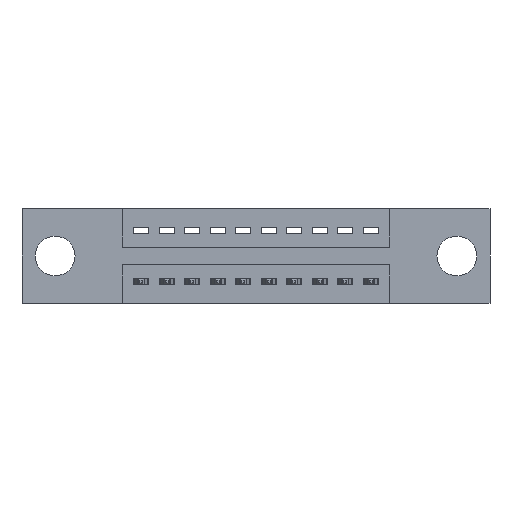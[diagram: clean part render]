
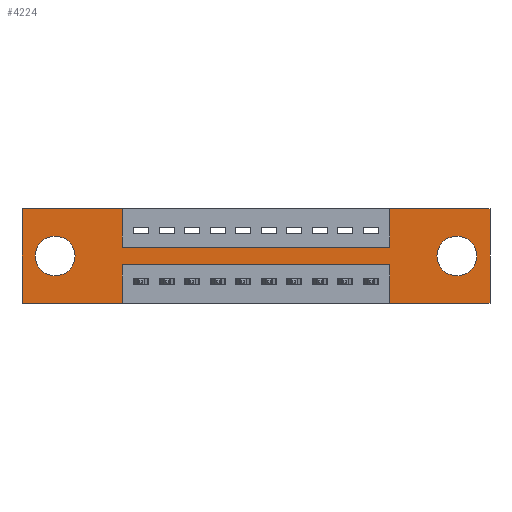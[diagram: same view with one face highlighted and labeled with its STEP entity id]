
A CAD part, front view. The second image highlights one B-rep face of the part: STEP entity #4224.
In plain terms, the highlighted planar face has unit normal (0, -1, 0).
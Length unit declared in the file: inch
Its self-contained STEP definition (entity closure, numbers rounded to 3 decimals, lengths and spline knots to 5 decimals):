
#251 = ORIENTED_EDGE ( 'NONE', *, *, #331, .F. ) ;
#302 = EDGE_CURVE ( 'NONE', #4691, #10908, #1327, .T. ) ;
#331 = EDGE_CURVE ( 'NONE', #7108, #2390, #3568, .T. ) ;
#503 = VECTOR ( 'NONE', #3563, 39.37008 ) ;
#579 = CARTESIAN_POINT ( 'NONE',  ( 0.3925, 0., -0.22 ) ) ;
#638 = CIRCLE ( 'NONE', #8570, 0.078 ) ;
#676 = EDGE_CURVE ( 'NONE', #3560, #1335, #5312, .T. ) ;
#864 = LINE ( 'NONE', #6454, #5596 ) ;
#876 = ORIENTED_EDGE ( 'NONE', *, *, #302, .T. ) ;
#935 = CARTESIAN_POINT ( 'NONE',  ( 0.13, 0., -0.185 ) ) ;
#1036 = VECTOR ( 'NONE', #4427, 39.37008 ) ;
#1044 = EDGE_CURVE ( 'NONE', #5193, #8139, #10566, .T. ) ;
#1082 = VECTOR ( 'NONE', #11482, 39.37008 ) ;
#1116 = EDGE_CURVE ( 'NONE', #2390, #2133, #864, .T. ) ;
#1207 = CIRCLE ( 'NONE', #10180, 0.078 ) ;
#1274 = FACE_BOUND ( 'NONE', #7116, .T. ) ;
#1327 = CIRCLE ( 'NONE', #3244, 0.078 ) ;
#1335 = VERTEX_POINT ( 'NONE', #3687 ) ;
#1365 = VECTOR ( 'NONE', #3258, 39.37008 ) ;
#1405 = DIRECTION ( 'NONE',  ( 0., 1., 0. ) ) ;
#1567 = FACE_BOUND ( 'NONE', #4058, .T. ) ;
#1664 = CARTESIAN_POINT ( 'NONE',  ( 1.835, 0., 0. ) ) ;
#1784 = CARTESIAN_POINT ( 'NONE',  ( 0.3925, 0., -0.15 ) ) ;
#1871 = DIRECTION ( 'NONE',  ( 0., 0., 1. ) ) ;
#2133 = VERTEX_POINT ( 'NONE', #1784 ) ;
#2157 = CARTESIAN_POINT ( 'NONE',  ( 0., 0., 0. ) ) ;
#2176 = CARTESIAN_POINT ( 'NONE',  ( 0., 0., 0. ) ) ;
#2212 = CARTESIAN_POINT ( 'NONE',  ( 0.3925, 0., -0.37 ) ) ;
#2390 = VERTEX_POINT ( 'NONE', #10811 ) ;
#2412 = EDGE_CURVE ( 'NONE', #10908, #4691, #8534, .T. ) ;
#2504 = ORIENTED_EDGE ( 'NONE', *, *, #10839, .F. ) ;
#2682 = VECTOR ( 'NONE', #3116, 39.37008 ) ;
#2815 = VECTOR ( 'NONE', #5090, 39.37008 ) ;
#2950 = ORIENTED_EDGE ( 'NONE', *, *, #1116, .F. ) ;
#2960 = VERTEX_POINT ( 'NONE', #6413 ) ;
#3116 = DIRECTION ( 'NONE',  ( 1., 0., 0. ) ) ;
#3244 = AXIS2_PLACEMENT_3D ( 'NONE', #4692, #5480, #7324 ) ;
#3258 = DIRECTION ( 'NONE',  ( 0., 0., 1. ) ) ;
#3499 = VERTEX_POINT ( 'NONE', #2212 ) ;
#3560 = VERTEX_POINT ( 'NONE', #1664 ) ;
#3563 = DIRECTION ( 'NONE',  ( 0., 0., -1. ) ) ;
#3568 = LINE ( 'NONE', #7369, #1036 ) ;
#3642 = LINE ( 'NONE', #3901, #503 ) ;
#3687 = CARTESIAN_POINT ( 'NONE',  ( 1.835, 0., -0.37 ) ) ;
#3814 = CARTESIAN_POINT ( 'NONE',  ( 0., 0., -0.37 ) ) ;
#3901 = CARTESIAN_POINT ( 'NONE',  ( 0.3925, 0., -0.37 ) ) ;
#4058 = EDGE_LOOP ( 'NONE', ( #5442, #4737 ) ) ;
#4097 = EDGE_CURVE ( 'NONE', #2133, #10636, #7401, .T. ) ;
#4150 = CARTESIAN_POINT ( 'NONE',  ( 0.3925, 0., -0.22 ) ) ;
#4224 = ADVANCED_FACE ( 'NONE', ( #1274, #1567, #5989 ), #11697, .T. ) ;
#4419 = CARTESIAN_POINT ( 'NONE',  ( 0., 0., -0.37 ) ) ;
#4427 = DIRECTION ( 'NONE',  ( 1., 0., 0. ) ) ;
#4543 = CARTESIAN_POINT ( 'NONE',  ( 0., 0., 0. ) ) ;
#4691 = VERTEX_POINT ( 'NONE', #5506 ) ;
#4692 = CARTESIAN_POINT ( 'NONE',  ( 1.705, 0., -0.185 ) ) ;
#4737 = ORIENTED_EDGE ( 'NONE', *, *, #8974, .T. ) ;
#4862 = EDGE_CURVE ( 'NONE', #8139, #3499, #3642, .T. ) ;
#4891 = ORIENTED_EDGE ( 'NONE', *, *, #5705, .F. ) ;
#5054 = LINE ( 'NONE', #2176, #7197 ) ;
#5090 = DIRECTION ( 'NONE',  ( 0., 0., -1. ) ) ;
#5138 = VERTEX_POINT ( 'NONE', #11431 ) ;
#5139 = CARTESIAN_POINT ( 'NONE',  ( 1.835, 0., 0. ) ) ;
#5193 = VERTEX_POINT ( 'NONE', #10328 ) ;
#5312 = LINE ( 'NONE', #5139, #2815 ) ;
#5442 = ORIENTED_EDGE ( 'NONE', *, *, #10729, .T. ) ;
#5480 = DIRECTION ( 'NONE',  ( 0., 1., 0. ) ) ;
#5506 = CARTESIAN_POINT ( 'NONE',  ( 1.705, 0., -0.263 ) ) ;
#5596 = VECTOR ( 'NONE', #8220, 39.37008 ) ;
#5705 = EDGE_CURVE ( 'NONE', #5138, #5193, #8170, .T. ) ;
#5772 = LINE ( 'NONE', #4419, #10203 ) ;
#5976 = EDGE_CURVE ( 'NONE', #1335, #5138, #7759, .T. ) ;
#5989 = FACE_OUTER_BOUND ( 'NONE', #8285, .T. ) ;
#5997 = CARTESIAN_POINT ( 'NONE',  ( 0.13, 0., -0.263 ) ) ;
#6000 = CARTESIAN_POINT ( 'NONE',  ( 1.705, 0., -0.107 ) ) ;
#6264 = VERTEX_POINT ( 'NONE', #5997 ) ;
#6266 = DIRECTION ( 'NONE',  ( 0., 0., -1. ) ) ;
#6413 = CARTESIAN_POINT ( 'NONE',  ( 1.4425, 0., 0. ) ) ;
#6454 = CARTESIAN_POINT ( 'NONE',  ( 0.3925, 0., 0. ) ) ;
#7016 = CARTESIAN_POINT ( 'NONE',  ( 0.13, 0., -0.185 ) ) ;
#7033 = EDGE_CURVE ( 'NONE', #3499, #7397, #5772, .T. ) ;
#7048 = CARTESIAN_POINT ( 'NONE',  ( 1.4425, 0., -0.15 ) ) ;
#7108 = VERTEX_POINT ( 'NONE', #4543 ) ;
#7116 = EDGE_LOOP ( 'NONE', ( #10989, #876 ) ) ;
#7197 = VECTOR ( 'NONE', #9475, 39.37008 ) ;
#7284 = ORIENTED_EDGE ( 'NONE', *, *, #1044, .F. ) ;
#7324 = DIRECTION ( 'NONE',  ( 0., 0., -1. ) ) ;
#7369 = CARTESIAN_POINT ( 'NONE',  ( 0., 0., 0. ) ) ;
#7397 = VERTEX_POINT ( 'NONE', #11087 ) ;
#7401 = LINE ( 'NONE', #11336, #11778 ) ;
#7459 = DIRECTION ( 'NONE',  ( 0., 1., 0. ) ) ;
#7759 = LINE ( 'NONE', #3814, #9823 ) ;
#7860 = VERTEX_POINT ( 'NONE', #9165 ) ;
#7879 = DIRECTION ( 'NONE',  ( 0., 0., 1. ) ) ;
#7896 = DIRECTION ( 'NONE',  ( 0., -1., 0. ) ) ;
#8139 = VERTEX_POINT ( 'NONE', #4150 ) ;
#8170 = LINE ( 'NONE', #10582, #1082 ) ;
#8220 = DIRECTION ( 'NONE',  ( 0., 0., -1. ) ) ;
#8238 = ORIENTED_EDGE ( 'NONE', *, *, #4862, .F. ) ;
#8249 = VECTOR ( 'NONE', #10741, 39.37008 ) ;
#8255 = CARTESIAN_POINT ( 'NONE',  ( 0., 0., -0.37 ) ) ;
#8285 = EDGE_LOOP ( 'NONE', ( #8238, #7284, #4891, #11680, #11421, #10039, #11136, #8811, #2950, #251, #2504, #8390 ) ) ;
#8390 = ORIENTED_EDGE ( 'NONE', *, *, #7033, .F. ) ;
#8456 = LINE ( 'NONE', #9647, #1365 ) ;
#8492 = AXIS2_PLACEMENT_3D ( 'NONE', #8255, #7896, #6266 ) ;
#8534 = CIRCLE ( 'NONE', #11546, 0.078 ) ;
#8570 = AXIS2_PLACEMENT_3D ( 'NONE', #7016, #1405, #7879 ) ;
#8811 = ORIENTED_EDGE ( 'NONE', *, *, #4097, .F. ) ;
#8974 = EDGE_CURVE ( 'NONE', #6264, #7860, #638, .T. ) ;
#9165 = CARTESIAN_POINT ( 'NONE',  ( 0.13, 0., -0.107 ) ) ;
#9475 = DIRECTION ( 'NONE',  ( 0., 0., 1. ) ) ;
#9496 = EDGE_CURVE ( 'NONE', #10636, #2960, #8456, .T. ) ;
#9647 = CARTESIAN_POINT ( 'NONE',  ( 1.4425, 0., 0. ) ) ;
#9768 = DIRECTION ( 'NONE',  ( -1., 0., 0. ) ) ;
#9823 = VECTOR ( 'NONE', #10919, 39.37008 ) ;
#9914 = LINE ( 'NONE', #2157, #2682 ) ;
#10039 = ORIENTED_EDGE ( 'NONE', *, *, #11494, .F. ) ;
#10180 = AXIS2_PLACEMENT_3D ( 'NONE', #935, #7459, #1871 ) ;
#10203 = VECTOR ( 'NONE', #9768, 39.37008 ) ;
#10328 = CARTESIAN_POINT ( 'NONE',  ( 1.4425, 0., -0.22 ) ) ;
#10566 = LINE ( 'NONE', #579, #8249 ) ;
#10582 = CARTESIAN_POINT ( 'NONE',  ( 1.4425, 0., -0.37 ) ) ;
#10636 = VERTEX_POINT ( 'NONE', #7048 ) ;
#10647 = DIRECTION ( 'NONE',  ( 0., 0., -1. ) ) ;
#10669 = DIRECTION ( 'NONE',  ( 0., 1., 0. ) ) ;
#10693 = CARTESIAN_POINT ( 'NONE',  ( 1.705, 0., -0.185 ) ) ;
#10729 = EDGE_CURVE ( 'NONE', #7860, #6264, #1207, .T. ) ;
#10741 = DIRECTION ( 'NONE',  ( -1., 0., 0. ) ) ;
#10811 = CARTESIAN_POINT ( 'NONE',  ( 0.3925, 0., 0. ) ) ;
#10839 = EDGE_CURVE ( 'NONE', #7397, #7108, #5054, .T. ) ;
#10908 = VERTEX_POINT ( 'NONE', #6000 ) ;
#10919 = DIRECTION ( 'NONE',  ( -1., 0., 0. ) ) ;
#10989 = ORIENTED_EDGE ( 'NONE', *, *, #2412, .T. ) ;
#11087 = CARTESIAN_POINT ( 'NONE',  ( 0., 0., -0.37 ) ) ;
#11136 = ORIENTED_EDGE ( 'NONE', *, *, #9496, .F. ) ;
#11336 = CARTESIAN_POINT ( 'NONE',  ( 0.3925, 0., -0.15 ) ) ;
#11361 = DIRECTION ( 'NONE',  ( 1., 0., 0. ) ) ;
#11421 = ORIENTED_EDGE ( 'NONE', *, *, #676, .F. ) ;
#11431 = CARTESIAN_POINT ( 'NONE',  ( 1.4425, 0., -0.37 ) ) ;
#11482 = DIRECTION ( 'NONE',  ( 0., 0., 1. ) ) ;
#11494 = EDGE_CURVE ( 'NONE', #2960, #3560, #9914, .T. ) ;
#11546 = AXIS2_PLACEMENT_3D ( 'NONE', #10693, #10669, #10647 ) ;
#11680 = ORIENTED_EDGE ( 'NONE', *, *, #5976, .F. ) ;
#11697 = PLANE ( 'NONE',  #8492 ) ;
#11778 = VECTOR ( 'NONE', #11361, 39.37008 ) ;
